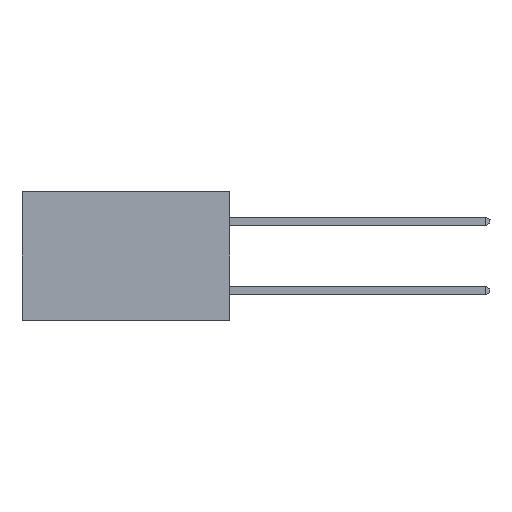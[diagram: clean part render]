
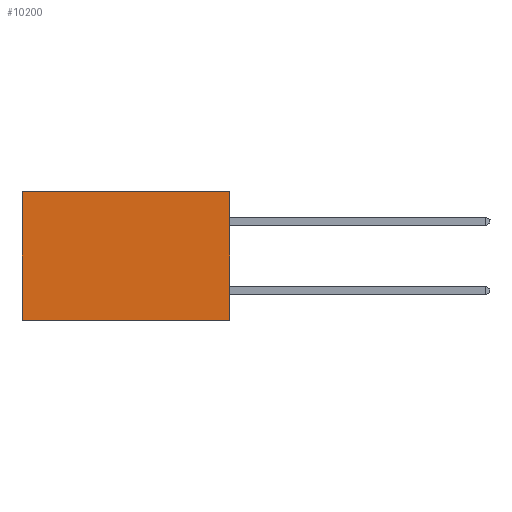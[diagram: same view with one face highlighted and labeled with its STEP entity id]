
A CAD part, left-side view. The second image highlights one B-rep face of the part: STEP entity #10200.
In plain terms, the highlighted planar face has unit normal (-1, 0, 0).
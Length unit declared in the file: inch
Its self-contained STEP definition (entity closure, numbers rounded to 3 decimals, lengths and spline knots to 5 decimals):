
#260 = LINE ( 'NONE', #2503, #9897 ) ;
#294 = CARTESIAN_POINT ( 'NONE',  ( 0.298, 0., 0. ) ) ;
#1294 = LINE ( 'NONE', #4193, #13776 ) ;
#1424 = DIRECTION ( 'NONE',  ( 1., 0., 0. ) ) ;
#2503 = CARTESIAN_POINT ( 'NONE',  ( 0.298, 0.6, 0. ) ) ;
#2532 = DIRECTION ( 'NONE',  ( 0., 0., -1. ) ) ;
#2786 = CARTESIAN_POINT ( 'NONE',  ( 0.298, 0., 0. ) ) ;
#2946 = EDGE_CURVE ( 'NONE', #11644, #13941, #1294, .T. ) ;
#3080 = LINE ( 'NONE', #8348, #13374 ) ;
#3593 = PLANE ( 'NONE',  #10952 ) ;
#3714 = ORIENTED_EDGE ( 'NONE', *, *, #12025, .T. ) ;
#4193 = CARTESIAN_POINT ( 'NONE',  ( 0.298, 0., 0. ) ) ;
#4478 = DIRECTION ( 'NONE',  ( 0., 0., -1. ) ) ;
#4583 = VERTEX_POINT ( 'NONE', #9980 ) ;
#5101 = DIRECTION ( 'NONE',  ( 0., 1., 0. ) ) ;
#6760 = VECTOR ( 'NONE', #4478, 39.37008 ) ;
#7028 = EDGE_LOOP ( 'NONE', ( #3714, #9615, #8785, #8143 ) ) ;
#7235 = FACE_OUTER_BOUND ( 'NONE', #7028, .T. ) ;
#8143 = ORIENTED_EDGE ( 'NONE', *, *, #2946, .T. ) ;
#8348 = CARTESIAN_POINT ( 'NONE',  ( 0.298, 0., -0.37 ) ) ;
#8746 = EDGE_CURVE ( 'NONE', #11644, #11303, #11851, .T. ) ;
#8785 = ORIENTED_EDGE ( 'NONE', *, *, #8746, .F. ) ;
#9615 = ORIENTED_EDGE ( 'NONE', *, *, #10937, .F. ) ;
#9897 = VECTOR ( 'NONE', #10163, 39.37008 ) ;
#9980 = CARTESIAN_POINT ( 'NONE',  ( 0.298, 0.6, -0.37 ) ) ;
#10163 = DIRECTION ( 'NONE',  ( 0., 0., -1. ) ) ;
#10200 = ADVANCED_FACE ( 'NONE', ( #7235 ), #3593, .F. ) ;
#10937 = EDGE_CURVE ( 'NONE', #11303, #4583, #3080, .T. ) ;
#10952 = AXIS2_PLACEMENT_3D ( 'NONE', #294, #1424, #2532 ) ;
#11303 = VERTEX_POINT ( 'NONE', #11654 ) ;
#11644 = VERTEX_POINT ( 'NONE', #2786 ) ;
#11654 = CARTESIAN_POINT ( 'NONE',  ( 0.298, 0., -0.37 ) ) ;
#11851 = LINE ( 'NONE', #11989, #6760 ) ;
#11989 = CARTESIAN_POINT ( 'NONE',  ( 0.298, 0., 0. ) ) ;
#12025 = EDGE_CURVE ( 'NONE', #13941, #4583, #260, .T. ) ;
#12402 = CARTESIAN_POINT ( 'NONE',  ( 0.298, 0.6, 0. ) ) ;
#13374 = VECTOR ( 'NONE', #5101, 39.37008 ) ;
#13776 = VECTOR ( 'NONE', #13835, 39.37008 ) ;
#13835 = DIRECTION ( 'NONE',  ( 0., 1., 0. ) ) ;
#13941 = VERTEX_POINT ( 'NONE', #12402 ) ;
